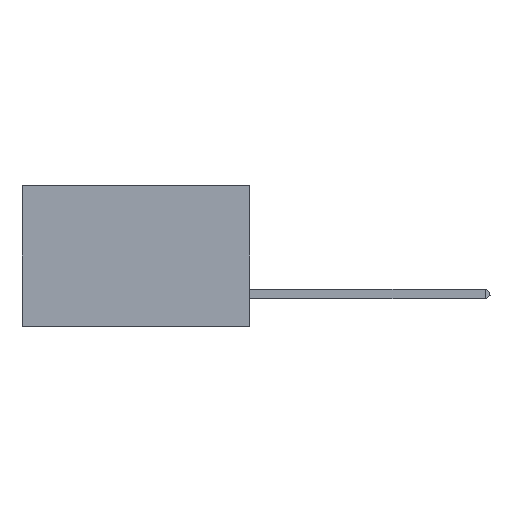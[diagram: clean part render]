
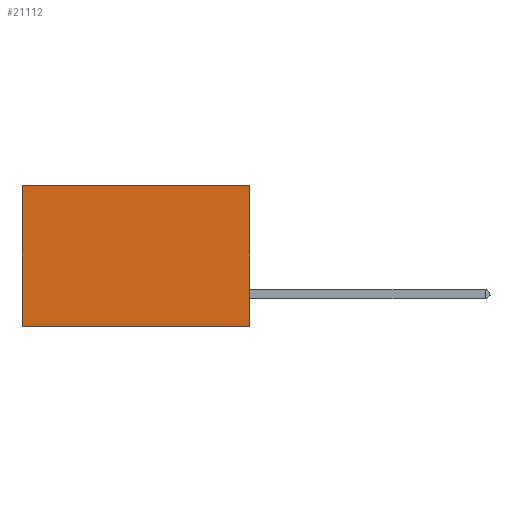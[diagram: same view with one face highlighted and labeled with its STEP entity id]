
A CAD part, left-side view. The second image highlights one B-rep face of the part: STEP entity #21112.
In plain terms, the highlighted planar face has unit normal (-1, 0, 0).
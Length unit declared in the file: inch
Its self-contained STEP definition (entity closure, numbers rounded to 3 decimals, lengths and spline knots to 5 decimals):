
#1305 = CARTESIAN_POINT ( 'NONE',  ( 0.2875, 0., 0. ) ) ;
#2544 = VERTEX_POINT ( 'NONE', #12248 ) ;
#2877 = CARTESIAN_POINT ( 'NONE',  ( 0.2875, 0., 0. ) ) ;
#3221 = LINE ( 'NONE', #2877, #20724 ) ;
#4383 = PLANE ( 'NONE',  #13205 ) ;
#4947 = LINE ( 'NONE', #14619, #6016 ) ;
#6016 = VECTOR ( 'NONE', #15689, 39.37008 ) ;
#6918 = EDGE_LOOP ( 'NONE', ( #14047, #17413, #22618, #21527 ) ) ;
#7010 = DIRECTION ( 'NONE',  ( 1., 0., 0. ) ) ;
#7095 = DIRECTION ( 'NONE',  ( 0., 0., -1. ) ) ;
#7992 = VERTEX_POINT ( 'NONE', #1305 ) ;
#8161 = VERTEX_POINT ( 'NONE', #12352 ) ;
#8522 = EDGE_CURVE ( 'NONE', #2544, #17031, #20694, .T. ) ;
#9245 = CARTESIAN_POINT ( 'NONE',  ( 0.2875, 0., 0. ) ) ;
#11374 = DIRECTION ( 'NONE',  ( 0., 0., -1. ) ) ;
#11855 = EDGE_CURVE ( 'NONE', #8161, #17031, #4947, .T. ) ;
#12046 = CARTESIAN_POINT ( 'NONE',  ( 0.2875, 0.6, -0.37 ) ) ;
#12248 = CARTESIAN_POINT ( 'NONE',  ( 0.2875, 0.6, 0. ) ) ;
#12352 = CARTESIAN_POINT ( 'NONE',  ( 0.2875, 0., -0.37 ) ) ;
#13205 = AXIS2_PLACEMENT_3D ( 'NONE', #9245, #7010, #11374 ) ;
#13546 = LINE ( 'NONE', #19377, #17122 ) ;
#14047 = ORIENTED_EDGE ( 'NONE', *, *, #8522, .T. ) ;
#14102 = DIRECTION ( 'NONE',  ( 0., 1., 0. ) ) ;
#14619 = CARTESIAN_POINT ( 'NONE',  ( 0.2875, 0., -0.37 ) ) ;
#15138 = DIRECTION ( 'NONE',  ( 0., 0., -1. ) ) ;
#15689 = DIRECTION ( 'NONE',  ( 0., 1., 0. ) ) ;
#17031 = VERTEX_POINT ( 'NONE', #12046 ) ;
#17122 = VECTOR ( 'NONE', #14102, 39.37008 ) ;
#17413 = ORIENTED_EDGE ( 'NONE', *, *, #11855, .F. ) ;
#19377 = CARTESIAN_POINT ( 'NONE',  ( 0.2875, 0., 0. ) ) ;
#20149 = VECTOR ( 'NONE', #7095, 39.37008 ) ;
#20694 = LINE ( 'NONE', #20869, #20149 ) ;
#20724 = VECTOR ( 'NONE', #15138, 39.37008 ) ;
#20840 = EDGE_CURVE ( 'NONE', #7992, #8161, #3221, .T. ) ;
#20869 = CARTESIAN_POINT ( 'NONE',  ( 0.2875, 0.6, 0. ) ) ;
#21112 = ADVANCED_FACE ( 'NONE', ( #21524 ), #4383, .F. ) ;
#21524 = FACE_OUTER_BOUND ( 'NONE', #6918, .T. ) ;
#21527 = ORIENTED_EDGE ( 'NONE', *, *, #22451, .T. ) ;
#22451 = EDGE_CURVE ( 'NONE', #7992, #2544, #13546, .T. ) ;
#22618 = ORIENTED_EDGE ( 'NONE', *, *, #20840, .F. ) ;
